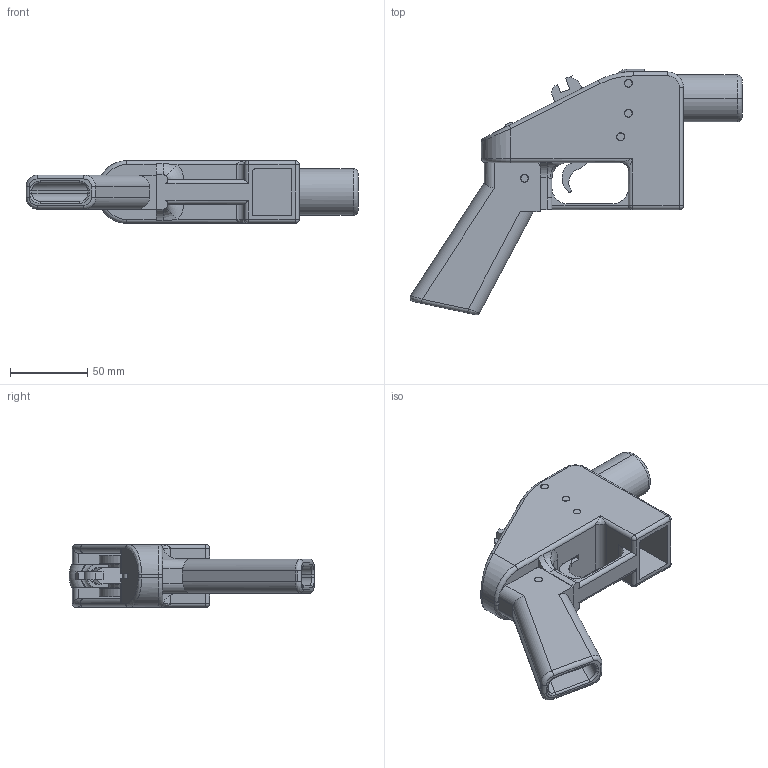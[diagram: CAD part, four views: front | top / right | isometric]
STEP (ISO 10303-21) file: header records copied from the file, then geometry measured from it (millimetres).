
FILE_DESCRIPTION (( 'STEP AP214' ), '1' );
FILE_NAME ('LiberatorSWNative.STEP', '2013-05-27T22:40:06', ( 'Asher' ), ( '' ), 'SwSTEP 2.0', 'SolidWorks 2013', '' );
FILE_SCHEMA (( 'AUTOMOTIVE_DESIGN' ));
Length unit declared in the file: millimetre
Products named in the file (16): hammer pin; trigger spring; HammerSpringAssem; spring connecting rod; spring connecting rod bushing; Spring; frame pins (x3); grip pin; firing pin bushing; GripRemodeled; trigger; hammer; 380 barrel (threaded); hammer body; frame (no sn); LiberatorSWNative
Assembly tree (18 placements, depth 3):
  LiberatorSWNative
    frame (no sn)
    hammer body
    380 barrel (threaded)
    hammer
    trigger
    GripRemodeled
    firing pin bushing
    grip pin
    frame pins (x3)  x3
    HammerSpringAssem
      Spring  x2
      spring connecting rod bushing
      spring connecting rod
    trigger spring
    hammer pin
Bounding box: 215.38 x 159.35 x 40.64 mm (x, y, z)
Volume: 298351.4 mm3; surface area: 102565.7 mm2
Topology: 17 solids, 17 shells, 519 faces, 1340 edges, 855 vertices
Faces by surface type: cylinder 222, plane 222, torus 47, bspline 20, cone 4, sphere 4
Entity records: 17283 total; most frequent: CARTESIAN_POINT 4241, DIRECTION 2679, ORIENTED_EDGE 2572, EDGE_CURVE 1286, AXIS2_PLACEMENT_3D 987, VERTEX_POINT 823, VECTOR 705, LINE 705
